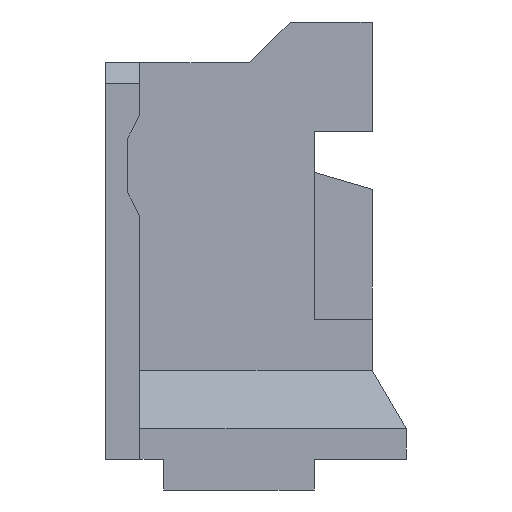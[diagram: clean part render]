
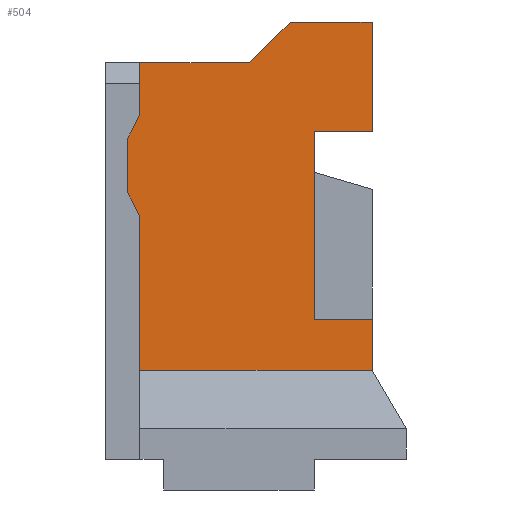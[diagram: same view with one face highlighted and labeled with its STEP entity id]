
A CAD part, left-side view. The second image highlights one B-rep face of the part: STEP entity #504.
In plain terms, the highlighted planar face has unit normal (-1, 0, 0).
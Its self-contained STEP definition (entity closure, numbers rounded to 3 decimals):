
#152 = EDGE_CURVE ( 'NONE', #5833, #5466, #9217, .T. ) ;
#323 = ORIENTED_EDGE ( 'NONE', *, *, #8389, .F. ) ;
#334 = EDGE_LOOP ( 'NONE', ( #7566, #323, #6271, #11503, #11911, #12267, #2326, #5565, #6080, #10049, #5017, #8943, #2027, #6926 ) ) ;
#362 = CARTESIAN_POINT ( 'NONE',  ( -1.25, 1.1, -0.75 ) ) ;
#369 = VERTEX_POINT ( 'NONE', #9440 ) ;
#394 = CARTESIAN_POINT ( 'NONE',  ( -1.25, 1.1, -4.5 ) ) ;
#412 = CARTESIAN_POINT ( 'NONE',  ( -1.25, -1.1, 0.6 ) ) ;
#504 = ADVANCED_FACE ( 'NONE', ( #2450 ), #9054, .F. ) ;
#510 = VERTEX_POINT ( 'NONE', #3163 ) ;
#598 = LINE ( 'NONE', #1400, #3807 ) ;
#664 = DIRECTION ( 'NONE',  ( 0., -0.707, 0.707 ) ) ;
#718 = CARTESIAN_POINT ( 'NONE',  ( -1.25, -2.3, 0.6 ) ) ;
#888 = CARTESIAN_POINT ( 'NONE',  ( -1.25, -1.45, -3.75 ) ) ;
#899 = VECTOR ( 'NONE', #9290, 1000. ) ;
#1203 = CARTESIAN_POINT ( 'NONE',  ( -1.25, 1.275, -1.1 ) ) ;
#1218 = EDGE_CURVE ( 'NONE', #5628, #3652, #598, .T. ) ;
#1400 = CARTESIAN_POINT ( 'NONE',  ( -1.25, 1.1, 0. ) ) ;
#1518 = EDGE_CURVE ( 'NONE', #369, #3065, #10721, .T. ) ;
#1697 = DIRECTION ( 'NONE',  ( 0., 0., -1. ) ) ;
#2027 = ORIENTED_EDGE ( 'NONE', *, *, #10178, .F. ) ;
#2035 = LINE ( 'NONE', #12383, #6364 ) ;
#2051 = CARTESIAN_POINT ( 'NONE',  ( -1.25, -2.3, -1. ) ) ;
#2326 = ORIENTED_EDGE ( 'NONE', *, *, #11245, .F. ) ;
#2346 = CARTESIAN_POINT ( 'NONE',  ( -1.25, 0., 0. ) ) ;
#2450 = FACE_OUTER_BOUND ( 'NONE', #334, .T. ) ;
#2573 = CARTESIAN_POINT ( 'NONE',  ( -1.25, 1.275, -1.9 ) ) ;
#2688 = EDGE_CURVE ( 'NONE', #8398, #4930, #6310, .T. ) ;
#2957 = DIRECTION ( 'NONE',  ( 0., 0., -1. ) ) ;
#2992 = DIRECTION ( 'NONE',  ( 0., 1., 0. ) ) ;
#3065 = VERTEX_POINT ( 'NONE', #9146 ) ;
#3163 = CARTESIAN_POINT ( 'NONE',  ( -1.25, -1.1, 0.6 ) ) ;
#3439 = CARTESIAN_POINT ( 'NONE',  ( -1.25, 3.057, -3.75 ) ) ;
#3611 = VERTEX_POINT ( 'NONE', #362 ) ;
#3652 = VERTEX_POINT ( 'NONE', #4354 ) ;
#3664 = EDGE_CURVE ( 'NONE', #5466, #5474, #4589, .T. ) ;
#3684 = DIRECTION ( 'NONE',  ( 0., 1., 0. ) ) ;
#3805 = VECTOR ( 'NONE', #10358, 1000. ) ;
#3807 = VECTOR ( 'NONE', #5274, 1000. ) ;
#4023 = CARTESIAN_POINT ( 'NONE',  ( -1.25, -1.45, -1. ) ) ;
#4190 = DIRECTION ( 'NONE',  ( 0., 0., -1. ) ) ;
#4246 = DIRECTION ( 'NONE',  ( 1., 0., 0. ) ) ;
#4256 = DIRECTION ( 'NONE',  ( 0., -0.447, 0.894 ) ) ;
#4266 = LINE ( 'NONE', #9182, #5031 ) ;
#4292 = VECTOR ( 'NONE', #2957, 1000. ) ;
#4354 = CARTESIAN_POINT ( 'NONE',  ( -1.25, -0.5, 0. ) ) ;
#4531 = CARTESIAN_POINT ( 'NONE',  ( -1.25, -2.3, -4.5 ) ) ;
#4589 = LINE ( 'NONE', #3439, #3805 ) ;
#4625 = AXIS2_PLACEMENT_3D ( 'NONE', #2346, #4246, #4190 ) ;
#4736 = LINE ( 'NONE', #12236, #5813 ) ;
#4810 = EDGE_CURVE ( 'NONE', #8069, #8398, #7769, .T. ) ;
#4924 = CARTESIAN_POINT ( 'NONE',  ( -1.25, 1.1, -2.25 ) ) ;
#4930 = VERTEX_POINT ( 'NONE', #4924 ) ;
#5017 = ORIENTED_EDGE ( 'NONE', *, *, #1518, .F. ) ;
#5031 = VECTOR ( 'NONE', #8237, 1000. ) ;
#5274 = DIRECTION ( 'NONE',  ( 0., -1., 0. ) ) ;
#5339 = CARTESIAN_POINT ( 'NONE',  ( -1.25, 1.275, -2.25 ) ) ;
#5349 = EDGE_CURVE ( 'NONE', #3611, #5628, #12120, .T. ) ;
#5466 = VERTEX_POINT ( 'NONE', #888 ) ;
#5474 = VERTEX_POINT ( 'NONE', #9860 ) ;
#5565 = ORIENTED_EDGE ( 'NONE', *, *, #3664, .F. ) ;
#5628 = VERTEX_POINT ( 'NONE', #7154 ) ;
#5697 = CARTESIAN_POINT ( 'NONE',  ( -1.25, 1.1, -5.8 ) ) ;
#5705 = DIRECTION ( 'NONE',  ( 0., 0., 1. ) ) ;
#5777 = DIRECTION ( 'NONE',  ( 0., 0., 1. ) ) ;
#5813 = VECTOR ( 'NONE', #4256, 1000. ) ;
#5833 = VERTEX_POINT ( 'NONE', #4023 ) ;
#5903 = CARTESIAN_POINT ( 'NONE',  ( -1.25, -1.45, -1. ) ) ;
#6080 = ORIENTED_EDGE ( 'NONE', *, *, #152, .F. ) ;
#6271 = ORIENTED_EDGE ( 'NONE', *, *, #9209, .F. ) ;
#6310 = LINE ( 'NONE', #5697, #6476 ) ;
#6364 = VECTOR ( 'NONE', #664, 1000. ) ;
#6476 = VECTOR ( 'NONE', #5777, 1000. ) ;
#6607 = LINE ( 'NONE', #412, #899 ) ;
#6663 = CARTESIAN_POINT ( 'NONE',  ( -1.25, 1.1, -5.8 ) ) ;
#6795 = CARTESIAN_POINT ( 'NONE',  ( -1.25, -3., -4.5 ) ) ;
#6926 = ORIENTED_EDGE ( 'NONE', *, *, #1218, .F. ) ;
#6930 = EDGE_CURVE ( 'NONE', #4930, #8589, #11531, .T. ) ;
#7154 = CARTESIAN_POINT ( 'NONE',  ( -1.25, 1.1, 0. ) ) ;
#7191 = VECTOR ( 'NONE', #2992, 1000. ) ;
#7566 = ORIENTED_EDGE ( 'NONE', *, *, #5349, .F. ) ;
#7769 = LINE ( 'NONE', #6795, #11912 ) ;
#7916 = EDGE_CURVE ( 'NONE', #510, #369, #6607, .T. ) ;
#8069 = VERTEX_POINT ( 'NONE', #4531 ) ;
#8237 = DIRECTION ( 'NONE',  ( 0., 0., -1. ) ) ;
#8241 = EDGE_CURVE ( 'NONE', #3065, #5833, #9652, .T. ) ;
#8273 = VECTOR ( 'NONE', #5705, 1000. ) ;
#8389 = EDGE_CURVE ( 'NONE', #12340, #3611, #4736, .T. ) ;
#8398 = VERTEX_POINT ( 'NONE', #394 ) ;
#8589 = VERTEX_POINT ( 'NONE', #2573 ) ;
#8943 = ORIENTED_EDGE ( 'NONE', *, *, #7916, .F. ) ;
#9054 = PLANE ( 'NONE',  #4625 ) ;
#9146 = CARTESIAN_POINT ( 'NONE',  ( -1.25, -2.3, -1. ) ) ;
#9182 = CARTESIAN_POINT ( 'NONE',  ( -1.25, -2.3, -1.85 ) ) ;
#9209 = EDGE_CURVE ( 'NONE', #8589, #12340, #12673, .T. ) ;
#9217 = LINE ( 'NONE', #5903, #4292 ) ;
#9290 = DIRECTION ( 'NONE',  ( 0., -1., 0. ) ) ;
#9440 = CARTESIAN_POINT ( 'NONE',  ( -1.25, -2.3, 0.6 ) ) ;
#9652 = LINE ( 'NONE', #2051, #7191 ) ;
#9783 = DIRECTION ( 'NONE',  ( 0., 0.447, 0.894 ) ) ;
#9797 = VECTOR ( 'NONE', #1697, 1000. ) ;
#9860 = CARTESIAN_POINT ( 'NONE',  ( -1.25, -2.3, -3.75 ) ) ;
#10049 = ORIENTED_EDGE ( 'NONE', *, *, #8241, .F. ) ;
#10178 = EDGE_CURVE ( 'NONE', #3652, #510, #2035, .T. ) ;
#10358 = DIRECTION ( 'NONE',  ( 0., -1., 0. ) ) ;
#10721 = LINE ( 'NONE', #718, #9797 ) ;
#11245 = EDGE_CURVE ( 'NONE', #5474, #8069, #4266, .T. ) ;
#11452 = VECTOR ( 'NONE', #12185, 1000. ) ;
#11503 = ORIENTED_EDGE ( 'NONE', *, *, #6930, .F. ) ;
#11531 = LINE ( 'NONE', #11784, #12606 ) ;
#11784 = CARTESIAN_POINT ( 'NONE',  ( -1.25, 1.1, -2.25 ) ) ;
#11911 = ORIENTED_EDGE ( 'NONE', *, *, #2688, .F. ) ;
#11912 = VECTOR ( 'NONE', #3684, 1000. ) ;
#12120 = LINE ( 'NONE', #6663, #8273 ) ;
#12185 = DIRECTION ( 'NONE',  ( 0., 0., 1. ) ) ;
#12236 = CARTESIAN_POINT ( 'NONE',  ( -1.25, 1.1, -0.75 ) ) ;
#12267 = ORIENTED_EDGE ( 'NONE', *, *, #4810, .F. ) ;
#12340 = VERTEX_POINT ( 'NONE', #1203 ) ;
#12383 = CARTESIAN_POINT ( 'NONE',  ( -1.25, -0.5, 0. ) ) ;
#12606 = VECTOR ( 'NONE', #9783, 1000. ) ;
#12673 = LINE ( 'NONE', #5339, #11452 ) ;
